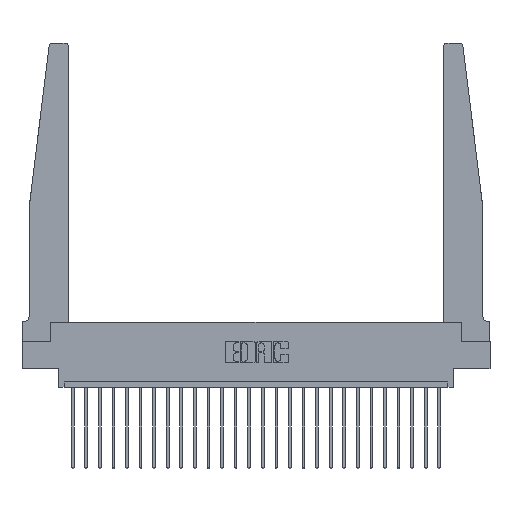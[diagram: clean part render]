
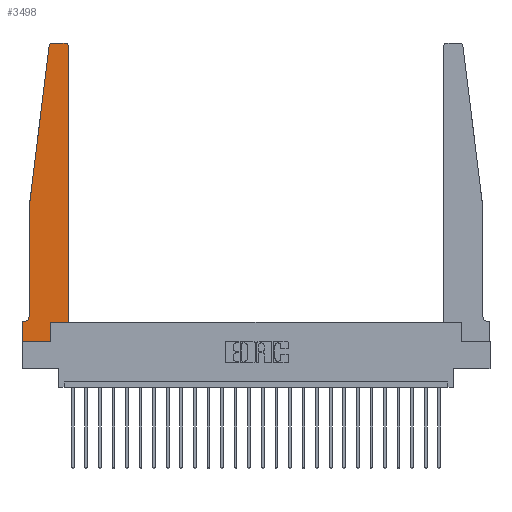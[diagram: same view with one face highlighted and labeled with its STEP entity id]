
A CAD part, top view. The second image highlights one B-rep face of the part: STEP entity #3498.
In plain terms, the highlighted planar face has unit normal (0, 0, 1).
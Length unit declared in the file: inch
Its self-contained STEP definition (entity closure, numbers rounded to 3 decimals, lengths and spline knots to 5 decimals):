
#129 = EDGE_CURVE ( 'NONE', #5383, #2880, #3698, .T. ) ;
#352 = EDGE_CURVE ( 'NONE', #2880, #12241, #22562, .T. ) ;
#486 = ORIENTED_EDGE ( 'NONE', *, *, #18544, .T. ) ;
#540 = CARTESIAN_POINT ( 'NONE',  ( 0.065, 0.1875, 0.37 ) ) ;
#1170 = DIRECTION ( 'NONE',  ( 0., 0., 1. ) ) ;
#1178 = LINE ( 'NONE', #2906, #16334 ) ;
#1490 = VECTOR ( 'NONE', #16069, 39.37008 ) ;
#1742 = EDGE_CURVE ( 'NONE', #5200, #21798, #19676, .T. ) ;
#1879 = CARTESIAN_POINT ( 'NONE',  ( 0.395, 2.72, 0.37 ) ) ;
#1949 = ORIENTED_EDGE ( 'NONE', *, *, #129, .T. ) ;
#1960 = CIRCLE ( 'NONE', #4379, 0.03 ) ;
#2144 = CARTESIAN_POINT ( 'NONE',  ( 0., 0., 0.37 ) ) ;
#2601 = VERTEX_POINT ( 'NONE', #9433 ) ;
#2880 = VERTEX_POINT ( 'NONE', #21978 ) ;
#2906 = CARTESIAN_POINT ( 'NONE',  ( 0., 0., 0.37 ) ) ;
#3160 = DIRECTION ( 'NONE',  ( 0., 0., -1. ) ) ;
#3498 = ADVANCED_FACE ( 'NONE', ( #7851 ), #17276, .T. ) ;
#3569 = CARTESIAN_POINT ( 'NONE',  ( 0.065, 1.25, 0.37 ) ) ;
#3698 = CIRCLE ( 'NONE', #14026, 0.03 ) ;
#4106 = VERTEX_POINT ( 'NONE', #15613 ) ;
#4379 = AXIS2_PLACEMENT_3D ( 'NONE', #14860, #1170, #12639 ) ;
#4502 = LINE ( 'NONE', #14215, #1490 ) ;
#4714 = CARTESIAN_POINT ( 'NONE',  ( 0.425, 0.18, 0.37 ) ) ;
#4918 = ORIENTED_EDGE ( 'NONE', *, *, #17658, .T. ) ;
#5115 = LINE ( 'NONE', #12705, #17915 ) ;
#5200 = VERTEX_POINT ( 'NONE', #3569 ) ;
#5292 = VERTEX_POINT ( 'NONE', #6309 ) ;
#5383 = VERTEX_POINT ( 'NONE', #21751 ) ;
#5636 = ORIENTED_EDGE ( 'NONE', *, *, #7831, .T. ) ;
#5790 = DIRECTION ( 'NONE',  ( -1., 0., 0. ) ) ;
#6309 = CARTESIAN_POINT ( 'NONE',  ( 0., 0., 0.37 ) ) ;
#6671 = EDGE_LOOP ( 'NONE', ( #10277, #22542, #5636, #24573, #486, #10315, #17291, #4918, #11391, #24274, #6800, #1949 ) ) ;
#6800 = ORIENTED_EDGE ( 'NONE', *, *, #14712, .T. ) ;
#7304 = VECTOR ( 'NONE', #19115, 39.37008 ) ;
#7831 = EDGE_CURVE ( 'NONE', #12017, #5200, #4502, .T. ) ;
#7851 = FACE_OUTER_BOUND ( 'NONE', #6671, .T. ) ;
#8096 = DIRECTION ( 'NONE',  ( 0., 0., 1. ) ) ;
#8560 = DIRECTION ( 'NONE',  ( 1., 0., 0. ) ) ;
#8724 = DIRECTION ( 'NONE',  ( 0., -1., 0. ) ) ;
#9433 = CARTESIAN_POINT ( 'NONE',  ( 0., 0.1875, 0.37 ) ) ;
#10277 = ORIENTED_EDGE ( 'NONE', *, *, #352, .T. ) ;
#10315 = ORIENTED_EDGE ( 'NONE', *, *, #17860, .T. ) ;
#10509 = EDGE_CURVE ( 'NONE', #12241, #12017, #1960, .T. ) ;
#11230 = VECTOR ( 'NONE', #13828, 39.37008 ) ;
#11391 = ORIENTED_EDGE ( 'NONE', *, *, #16988, .T. ) ;
#11405 = LINE ( 'NONE', #16870, #13205 ) ;
#11518 = LINE ( 'NONE', #2144, #7304 ) ;
#12017 = VERTEX_POINT ( 'NONE', #22915 ) ;
#12241 = VERTEX_POINT ( 'NONE', #21911 ) ;
#12639 = DIRECTION ( 'NONE',  ( 1., 0., 0. ) ) ;
#12705 = CARTESIAN_POINT ( 'NONE',  ( 0.2605, 0.18, 0.37 ) ) ;
#12959 = CARTESIAN_POINT ( 'NONE',  ( 0.015, 0.1875, 0.37 ) ) ;
#13090 = DIRECTION ( 'NONE',  ( -1., 0., 0. ) ) ;
#13205 = VECTOR ( 'NONE', #18499, 39.37008 ) ;
#13581 = VECTOR ( 'NONE', #5790, 39.37008 ) ;
#13828 = DIRECTION ( 'NONE',  ( 0., 1., 0. ) ) ;
#14026 = AXIS2_PLACEMENT_3D ( 'NONE', #1879, #15208, #17819 ) ;
#14137 = EDGE_CURVE ( 'NONE', #19544, #15356, #11405, .T. ) ;
#14215 = CARTESIAN_POINT ( 'NONE',  ( 0.065, 1.25, 0.37 ) ) ;
#14712 = EDGE_CURVE ( 'NONE', #15356, #5383, #23286, .T. ) ;
#14860 = CARTESIAN_POINT ( 'NONE',  ( 0.27653, 2.72, 0.37 ) ) ;
#15208 = DIRECTION ( 'NONE',  ( 0., 0., 1. ) ) ;
#15356 = VERTEX_POINT ( 'NONE', #22505 ) ;
#15613 = CARTESIAN_POINT ( 'NONE',  ( 0.2605, 0., 0.37 ) ) ;
#15694 = AXIS2_PLACEMENT_3D ( 'NONE', #19407, #8096, #19528 ) ;
#16069 = DIRECTION ( 'NONE',  ( -0.122, -0.992, 0. ) ) ;
#16334 = VECTOR ( 'NONE', #8560, 39.37008 ) ;
#16870 = CARTESIAN_POINT ( 'NONE',  ( 0.425, 0.18, 0.37 ) ) ;
#16988 = EDGE_CURVE ( 'NONE', #4106, #19544, #5115, .T. ) ;
#17058 = VERTEX_POINT ( 'NONE', #12959 ) ;
#17276 = PLANE ( 'NONE',  #15694 ) ;
#17291 = ORIENTED_EDGE ( 'NONE', *, *, #19593, .T. ) ;
#17658 = EDGE_CURVE ( 'NONE', #5292, #4106, #1178, .T. ) ;
#17819 = DIRECTION ( 'NONE',  ( 1., 0., 0. ) ) ;
#17860 = EDGE_CURVE ( 'NONE', #17058, #2601, #19230, .T. ) ;
#17915 = VECTOR ( 'NONE', #23782, 39.37008 ) ;
#18250 = DIRECTION ( 'NONE',  ( -1., 0., 0. ) ) ;
#18499 = DIRECTION ( 'NONE',  ( 1., 0., 0. ) ) ;
#18544 = EDGE_CURVE ( 'NONE', #21798, #17058, #22755, .T. ) ;
#18811 = CARTESIAN_POINT ( 'NONE',  ( 0.25, 2.75, 0.37 ) ) ;
#19115 = DIRECTION ( 'NONE',  ( 0., -1., 0. ) ) ;
#19178 = AXIS2_PLACEMENT_3D ( 'NONE', #21393, #3160, #18250 ) ;
#19230 = LINE ( 'NONE', #540, #13581 ) ;
#19407 = CARTESIAN_POINT ( 'NONE',  ( 0., 0.1875, 0.37 ) ) ;
#19528 = DIRECTION ( 'NONE',  ( 1., 0., 0. ) ) ;
#19544 = VERTEX_POINT ( 'NONE', #21492 ) ;
#19593 = EDGE_CURVE ( 'NONE', #2601, #5292, #11518, .T. ) ;
#19676 = LINE ( 'NONE', #23398, #24245 ) ;
#21393 = CARTESIAN_POINT ( 'NONE',  ( 0.015, 0.2375, 0.37 ) ) ;
#21492 = CARTESIAN_POINT ( 'NONE',  ( 0.2605, 0.18, 0.37 ) ) ;
#21751 = CARTESIAN_POINT ( 'NONE',  ( 0.425, 2.72, 0.37 ) ) ;
#21798 = VERTEX_POINT ( 'NONE', #22541 ) ;
#21911 = CARTESIAN_POINT ( 'NONE',  ( 0.27653, 2.75, 0.37 ) ) ;
#21978 = CARTESIAN_POINT ( 'NONE',  ( 0.395, 2.75, 0.37 ) ) ;
#22020 = VECTOR ( 'NONE', #13090, 39.37008 ) ;
#22505 = CARTESIAN_POINT ( 'NONE',  ( 0.425, 0.18, 0.37 ) ) ;
#22541 = CARTESIAN_POINT ( 'NONE',  ( 0.065, 0.2375, 0.37 ) ) ;
#22542 = ORIENTED_EDGE ( 'NONE', *, *, #10509, .T. ) ;
#22562 = LINE ( 'NONE', #18811, #22020 ) ;
#22755 = CIRCLE ( 'NONE', #19178, 0.05 ) ;
#22915 = CARTESIAN_POINT ( 'NONE',  ( 0.24675, 2.72367, 0.37 ) ) ;
#23286 = LINE ( 'NONE', #4714, #11230 ) ;
#23398 = CARTESIAN_POINT ( 'NONE',  ( 0.065, 1.25, 0.37 ) ) ;
#23782 = DIRECTION ( 'NONE',  ( 0., 1., 0. ) ) ;
#24245 = VECTOR ( 'NONE', #8724, 39.37008 ) ;
#24274 = ORIENTED_EDGE ( 'NONE', *, *, #14137, .T. ) ;
#24573 = ORIENTED_EDGE ( 'NONE', *, *, #1742, .T. ) ;
